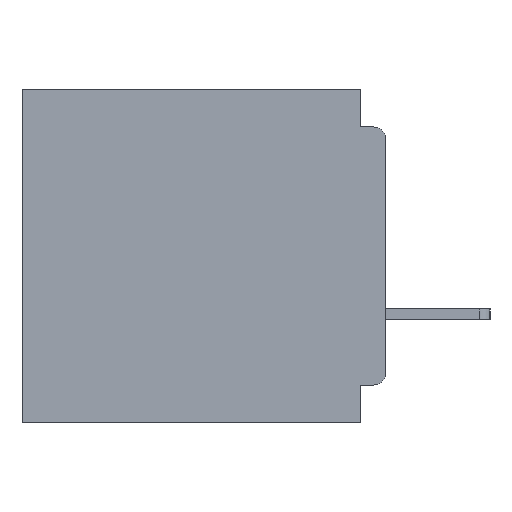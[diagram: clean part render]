
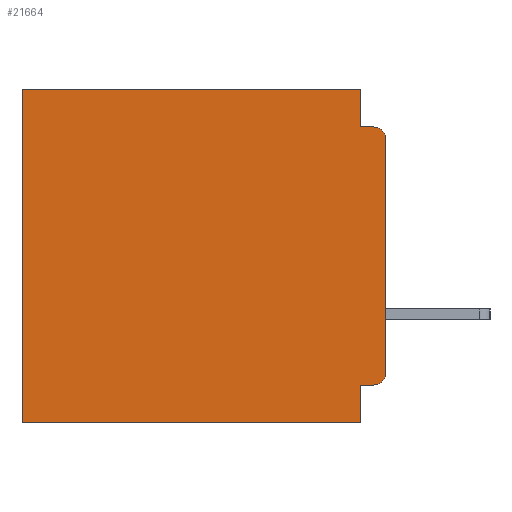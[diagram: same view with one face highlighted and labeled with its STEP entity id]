
A CAD part, left-side view. The second image highlights one B-rep face of the part: STEP entity #21664.
In plain terms, the highlighted planar face has unit normal (-1, 0, 0).
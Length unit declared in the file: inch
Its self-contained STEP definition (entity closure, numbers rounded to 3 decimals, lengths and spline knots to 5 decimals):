
#106 = EDGE_CURVE ( 'NONE', #21612, #23421, #44619, .T. ) ;
#1789 = DIRECTION ( 'NONE',  ( 0., 0., -1. ) ) ;
#1990 = ORIENTED_EDGE ( 'NONE', *, *, #14413, .T. ) ;
#2856 = EDGE_CURVE ( 'NONE', #23421, #10120, #47964, .T. ) ;
#3679 = VERTEX_POINT ( 'NONE', #5615 ) ;
#4008 = EDGE_CURVE ( 'NONE', #15997, #11889, #28790, .T. ) ;
#5615 = CARTESIAN_POINT ( 'NONE',  ( 0.3, 0.015, -0.045 ) ) ;
#5651 = ORIENTED_EDGE ( 'NONE', *, *, #37540, .F. ) ;
#6276 = VERTEX_POINT ( 'NONE', #15246 ) ;
#6471 = CARTESIAN_POINT ( 'NONE',  ( 0.3, 0., -0.4 ) ) ;
#7024 = CARTESIAN_POINT ( 'NONE',  ( 0.3, 0., -0.4 ) ) ;
#8091 = DIRECTION ( 'NONE',  ( -1., 0., 0. ) ) ;
#10120 = VERTEX_POINT ( 'NONE', #21303 ) ;
#11889 = VERTEX_POINT ( 'NONE', #16740 ) ;
#12075 = DIRECTION ( 'NONE',  ( 0., 1., 0. ) ) ;
#14413 = EDGE_CURVE ( 'NONE', #6276, #10120, #34289, .T. ) ;
#14756 = DIRECTION ( 'NONE',  ( 0., 0., -1. ) ) ;
#15246 = CARTESIAN_POINT ( 'NONE',  ( 0.3, 0.437, 0. ) ) ;
#15997 = VERTEX_POINT ( 'NONE', #48840 ) ;
#16590 = CARTESIAN_POINT ( 'NONE',  ( 0.3, 0., -0.4 ) ) ;
#16676 = DIRECTION ( 'NONE',  ( 0., -1., 0. ) ) ;
#16740 = CARTESIAN_POINT ( 'NONE',  ( 0.3, 0.031, -0.045 ) ) ;
#16959 = ORIENTED_EDGE ( 'NONE', *, *, #17784, .T. ) ;
#17127 = CARTESIAN_POINT ( 'NONE',  ( 0.3, 0.031, -0.4 ) ) ;
#17385 = FACE_OUTER_BOUND ( 'NONE', #50436, .T. ) ;
#17406 = VERTEX_POINT ( 'NONE', #36530 ) ;
#17784 = EDGE_CURVE ( 'NONE', #28086, #17406, #18593, .T. ) ;
#18235 = VECTOR ( 'NONE', #1789, 39.37008 ) ;
#18593 = CIRCLE ( 'NONE', #41196, 0.015 ) ;
#18754 = DIRECTION ( 'NONE',  ( 0., 0., -1. ) ) ;
#20385 = DIRECTION ( 'NONE',  ( -1., 0., 0. ) ) ;
#20543 = VECTOR ( 'NONE', #21547, 39.37008 ) ;
#20995 = EDGE_CURVE ( 'NONE', #27419, #17406, #57532, .T. ) ;
#21303 = CARTESIAN_POINT ( 'NONE',  ( 0.3, 0.437, -0.4 ) ) ;
#21441 = AXIS2_PLACEMENT_3D ( 'NONE', #7024, #54701, #26339 ) ;
#21517 = VECTOR ( 'NONE', #14756, 39.37008 ) ;
#21547 = DIRECTION ( 'NONE',  ( 0., 1., 0. ) ) ;
#21612 = VERTEX_POINT ( 'NONE', #40032 ) ;
#21664 = ADVANCED_FACE ( 'NONE', ( #17385 ), #49961, .F. ) ;
#22035 = LINE ( 'NONE', #59423, #20543 ) ;
#22323 = ORIENTED_EDGE ( 'NONE', *, *, #2856, .F. ) ;
#23230 = CARTESIAN_POINT ( 'NONE',  ( 0.3, 0.031, -0.4 ) ) ;
#23248 = DIRECTION ( 'NONE',  ( 0., 1., 0. ) ) ;
#23421 = VERTEX_POINT ( 'NONE', #17127 ) ;
#26339 = DIRECTION ( 'NONE',  ( 0., 0., -1. ) ) ;
#27419 = VERTEX_POINT ( 'NONE', #32934 ) ;
#28086 = VERTEX_POINT ( 'NONE', #47463 ) ;
#28790 = LINE ( 'NONE', #60042, #52429 ) ;
#29328 = ORIENTED_EDGE ( 'NONE', *, *, #40236, .T. ) ;
#32105 = VECTOR ( 'NONE', #18754, 39.37008 ) ;
#32182 = ORIENTED_EDGE ( 'NONE', *, *, #37964, .T. ) ;
#32373 = LINE ( 'NONE', #59144, #33853 ) ;
#32934 = CARTESIAN_POINT ( 'NONE',  ( 0.3, 0., -0.06 ) ) ;
#33267 = VECTOR ( 'NONE', #23248, 39.37008 ) ;
#33330 = ORIENTED_EDGE ( 'NONE', *, *, #20995, .F. ) ;
#33460 = EDGE_CURVE ( 'NONE', #11889, #3679, #32373, .T. ) ;
#33853 = VECTOR ( 'NONE', #16676, 39.37008 ) ;
#34289 = LINE ( 'NONE', #48066, #21517 ) ;
#35413 = VECTOR ( 'NONE', #12075, 39.37008 ) ;
#36530 = CARTESIAN_POINT ( 'NONE',  ( 0.3, 0., -0.34 ) ) ;
#36797 = CARTESIAN_POINT ( 'NONE',  ( 0.3, 0.015, -0.06 ) ) ;
#37540 = EDGE_CURVE ( 'NONE', #28086, #21612, #22035, .T. ) ;
#37964 = EDGE_CURVE ( 'NONE', #15997, #6276, #56795, .T. ) ;
#38660 = AXIS2_PLACEMENT_3D ( 'NONE', #36797, #8091, #41483 ) ;
#40032 = CARTESIAN_POINT ( 'NONE',  ( 0.3, 0.031, -0.355 ) ) ;
#40236 = EDGE_CURVE ( 'NONE', #27419, #3679, #45545, .T. ) ;
#41196 = AXIS2_PLACEMENT_3D ( 'NONE', #48852, #20385, #53602 ) ;
#41483 = DIRECTION ( 'NONE',  ( 0., 0., -1. ) ) ;
#44619 = LINE ( 'NONE', #23230, #32105 ) ;
#45545 = CIRCLE ( 'NONE', #38660, 0.015 ) ;
#45911 = ORIENTED_EDGE ( 'NONE', *, *, #33460, .F. ) ;
#47463 = CARTESIAN_POINT ( 'NONE',  ( 0.3, 0.015, -0.355 ) ) ;
#47964 = LINE ( 'NONE', #16590, #35413 ) ;
#48066 = CARTESIAN_POINT ( 'NONE',  ( 0.3, 0.437, -0.4 ) ) ;
#48840 = CARTESIAN_POINT ( 'NONE',  ( 0.3, 0.031, 0. ) ) ;
#48852 = CARTESIAN_POINT ( 'NONE',  ( 0.3, 0.015, -0.34 ) ) ;
#49752 = ORIENTED_EDGE ( 'NONE', *, *, #106, .F. ) ;
#49961 = PLANE ( 'NONE',  #21441 ) ;
#50436 = EDGE_LOOP ( 'NONE', ( #33330, #29328, #45911, #58076, #32182, #1990, #22323, #49752, #5651, #16959 ) ) ;
#52429 = VECTOR ( 'NONE', #60391, 39.37008 ) ;
#53602 = DIRECTION ( 'NONE',  ( 0., 0., -1. ) ) ;
#54701 = DIRECTION ( 'NONE',  ( 1., 0., 0. ) ) ;
#56407 = CARTESIAN_POINT ( 'NONE',  ( 0.3, 0., 0. ) ) ;
#56795 = LINE ( 'NONE', #56407, #33267 ) ;
#57532 = LINE ( 'NONE', #6471, #18235 ) ;
#58076 = ORIENTED_EDGE ( 'NONE', *, *, #4008, .F. ) ;
#59144 = CARTESIAN_POINT ( 'NONE',  ( 0.3, 0., -0.045 ) ) ;
#59423 = CARTESIAN_POINT ( 'NONE',  ( 0.3, 0., -0.355 ) ) ;
#60042 = CARTESIAN_POINT ( 'NONE',  ( 0.3, 0.031, 0. ) ) ;
#60391 = DIRECTION ( 'NONE',  ( 0., 0., -1. ) ) ;
